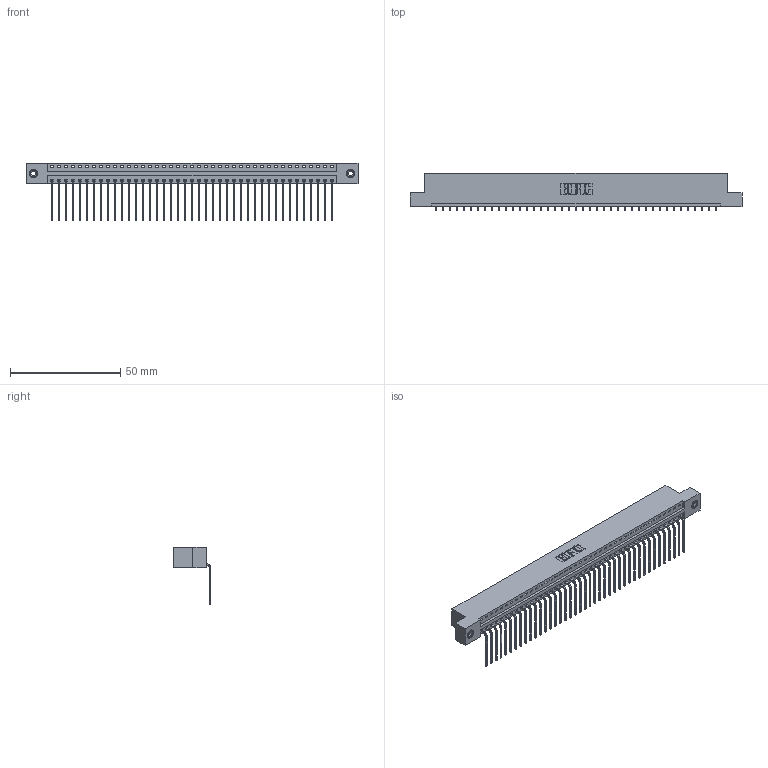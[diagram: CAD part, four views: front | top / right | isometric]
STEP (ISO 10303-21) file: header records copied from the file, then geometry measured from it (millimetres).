
FILE_DESCRIPTION (( 'STEP AP203' ), '1' );
FILE_NAME ('396-041-559-108.STEP', '2019-10-31T22:50:25', ( '' ), ( '' ), 'SwSTEP 2.0', 'SolidWorks 2016', '' );
FILE_SCHEMA (( 'CONFIG_CONTROL_DESIGN' ));
Length unit declared in the file: inch
Products named in the file (4): 396-041-559-108; 346 Part_Flush Mounting Lugs - 0.156 Dia-TI; 345-292-001_558 559 Tail - 1; 345-250-001_345-250-003-102
Assembly tree (44 placements, depth 2):
  396-041-559-108
    346 Part_Flush Mounting Lugs - 0.156 Dia-TI
    345-292-001_558 559 Tail - 1  x41
    345-250-001_345-250-003-102  x2
Bounding box: 150.75 x 17.08 x 26.16 mm (x, y, z)
Volume: 14553.2 mm3; surface area: 19015.6 mm2
Topology: 44 solids, 44 shells, 2642 faces, 7927 edges, 5222 vertices
Faces by surface type: plane 1830, cylinder 796, cone 12, torus 4
Entity records: 26850 total; most frequent: CARTESIAN_POINT 4586, ORIENTED_EDGE 4554, DIRECTION 4073, EDGE_CURVE 2277, VECTOR 1961, LINE 1961, VERTEX_POINT 1512, AXIS2_PLACEMENT_3D 1056
